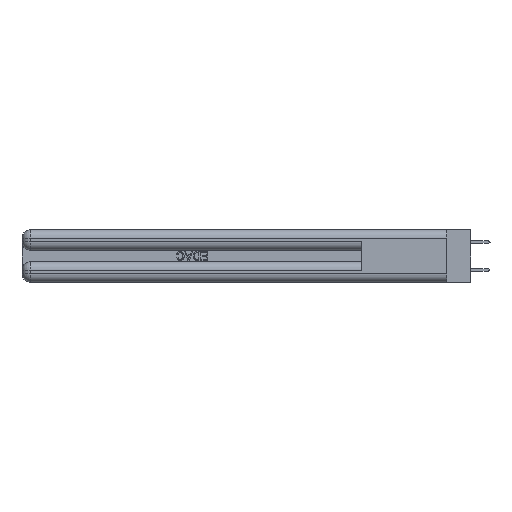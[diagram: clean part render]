
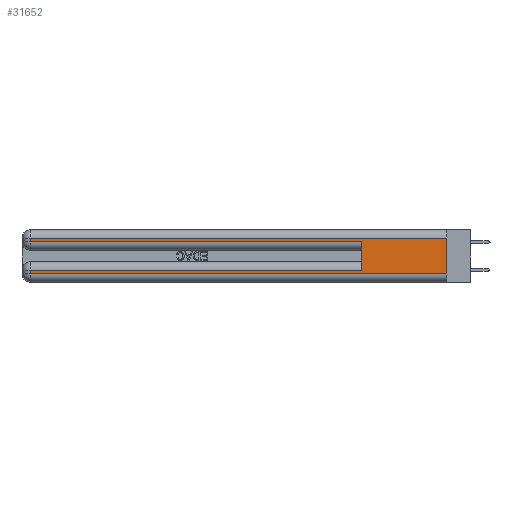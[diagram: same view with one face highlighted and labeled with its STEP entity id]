
A CAD part, left-side view. The second image highlights one B-rep face of the part: STEP entity #31652.
In plain terms, the highlighted planar face has unit normal (-1, 0, 0).
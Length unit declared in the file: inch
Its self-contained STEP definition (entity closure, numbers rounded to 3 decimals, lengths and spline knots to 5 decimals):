
#343 = ORIENTED_EDGE ( 'NONE', *, *, #30848, .F. ) ;
#683 = LINE ( 'NONE', #21270, #17257 ) ;
#4552 = LINE ( 'NONE', #17700, #21272 ) ;
#4769 = CARTESIAN_POINT ( 'NONE',  ( 0., 2.94, 0.085 ) ) ;
#5385 = CARTESIAN_POINT ( 'NONE',  ( 0., 0., 0.31 ) ) ;
#5494 = LINE ( 'NONE', #15968, #21512 ) ;
#5764 = VECTOR ( 'NONE', #12237, 39.37008 ) ;
#6952 = CARTESIAN_POINT ( 'NONE',  ( 0., 0., 0.37 ) ) ;
#9309 = VERTEX_POINT ( 'NONE', #21858 ) ;
#11078 = VERTEX_POINT ( 'NONE', #4769 ) ;
#12237 = DIRECTION ( 'NONE',  ( 0., -1., 0. ) ) ;
#12829 = EDGE_CURVE ( 'NONE', #11078, #34308, #37535, .T. ) ;
#13112 = FACE_OUTER_BOUND ( 'NONE', #19970, .T. ) ;
#13216 = DIRECTION ( 'NONE',  ( 0., 0., -1. ) ) ;
#13638 = VECTOR ( 'NONE', #13782, 39.37008 ) ;
#13782 = DIRECTION ( 'NONE',  ( 0., 0., -1. ) ) ;
#15032 = EDGE_CURVE ( 'NONE', #41179, #26382, #5494, .T. ) ;
#15567 = LINE ( 'NONE', #33502, #36997 ) ;
#15751 = EDGE_CURVE ( 'NONE', #24305, #9309, #39404, .T. ) ;
#15910 = VERTEX_POINT ( 'NONE', #30219 ) ;
#15968 = CARTESIAN_POINT ( 'NONE',  ( 0., 0.6, 0.145 ) ) ;
#16238 = DIRECTION ( 'NONE',  ( 0., 1., 0. ) ) ;
#17257 = VECTOR ( 'NONE', #42311, 39.37008 ) ;
#17700 = CARTESIAN_POINT ( 'NONE',  ( 0., 0., 0.06 ) ) ;
#19772 = DIRECTION ( 'NONE',  ( 0., 0., 1. ) ) ;
#19970 = EDGE_LOOP ( 'NONE', ( #343, #23548, #22798, #26277, #27971, #21945, #26931, #32576 ) ) ;
#20023 = PLANE ( 'NONE',  #31714 ) ;
#21270 = CARTESIAN_POINT ( 'NONE',  ( 0., 2.94, 0.37 ) ) ;
#21272 = VECTOR ( 'NONE', #32093, 39.37008 ) ;
#21512 = VECTOR ( 'NONE', #19772, 39.37008 ) ;
#21858 = CARTESIAN_POINT ( 'NONE',  ( 0., 2.94, 0.31 ) ) ;
#21945 = ORIENTED_EDGE ( 'NONE', *, *, #22672, .T. ) ;
#22627 = CARTESIAN_POINT ( 'NONE',  ( 0., 0.6, 0.285 ) ) ;
#22672 = EDGE_CURVE ( 'NONE', #41179, #11078, #15567, .T. ) ;
#22738 = LINE ( 'NONE', #36407, #5764 ) ;
#22798 = ORIENTED_EDGE ( 'NONE', *, *, #40234, .T. ) ;
#23172 = DIRECTION ( 'NONE',  ( 0., 0., -1. ) ) ;
#23272 = LINE ( 'NONE', #6952, #35977 ) ;
#23377 = EDGE_CURVE ( 'NONE', #34308, #34762, #4552, .T. ) ;
#23548 = ORIENTED_EDGE ( 'NONE', *, *, #15751, .T. ) ;
#24305 = VERTEX_POINT ( 'NONE', #35025 ) ;
#26197 = DIRECTION ( 'NONE',  ( 0., 1., 0. ) ) ;
#26277 = ORIENTED_EDGE ( 'NONE', *, *, #38271, .T. ) ;
#26382 = VERTEX_POINT ( 'NONE', #22627 ) ;
#26931 = ORIENTED_EDGE ( 'NONE', *, *, #12829, .T. ) ;
#27891 = CARTESIAN_POINT ( 'NONE',  ( 0., 0.6, 0.085 ) ) ;
#27971 = ORIENTED_EDGE ( 'NONE', *, *, #15032, .F. ) ;
#29413 = CARTESIAN_POINT ( 'NONE',  ( 0., 2.94, 0.06 ) ) ;
#29449 = VECTOR ( 'NONE', #26197, 39.37008 ) ;
#30219 = CARTESIAN_POINT ( 'NONE',  ( 0., 2.94, 0.285 ) ) ;
#30848 = EDGE_CURVE ( 'NONE', #24305, #34762, #23272, .T. ) ;
#31652 = ADVANCED_FACE ( 'NONE', ( #13112 ), #20023, .F. ) ;
#31714 = AXIS2_PLACEMENT_3D ( 'NONE', #37284, #33712, #23172 ) ;
#32093 = DIRECTION ( 'NONE',  ( 0., -1., 0. ) ) ;
#32576 = ORIENTED_EDGE ( 'NONE', *, *, #23377, .T. ) ;
#32874 = CARTESIAN_POINT ( 'NONE',  ( 0., 0., 0.06 ) ) ;
#33502 = CARTESIAN_POINT ( 'NONE',  ( 0., 0., 0.085 ) ) ;
#33712 = DIRECTION ( 'NONE',  ( 1., 0., 0. ) ) ;
#34308 = VERTEX_POINT ( 'NONE', #29413 ) ;
#34762 = VERTEX_POINT ( 'NONE', #32874 ) ;
#35025 = CARTESIAN_POINT ( 'NONE',  ( 0., 0., 0.31 ) ) ;
#35977 = VECTOR ( 'NONE', #13216, 39.37008 ) ;
#36407 = CARTESIAN_POINT ( 'NONE',  ( 0., 0., 0.285 ) ) ;
#36997 = VECTOR ( 'NONE', #16238, 39.37008 ) ;
#37284 = CARTESIAN_POINT ( 'NONE',  ( 0., 0., 0.37 ) ) ;
#37535 = LINE ( 'NONE', #43554, #13638 ) ;
#38271 = EDGE_CURVE ( 'NONE', #15910, #26382, #22738, .T. ) ;
#39404 = LINE ( 'NONE', #5385, #29449 ) ;
#40234 = EDGE_CURVE ( 'NONE', #9309, #15910, #683, .T. ) ;
#41179 = VERTEX_POINT ( 'NONE', #27891 ) ;
#42311 = DIRECTION ( 'NONE',  ( 0., 0., -1. ) ) ;
#43554 = CARTESIAN_POINT ( 'NONE',  ( 0., 2.94, 0.37 ) ) ;
